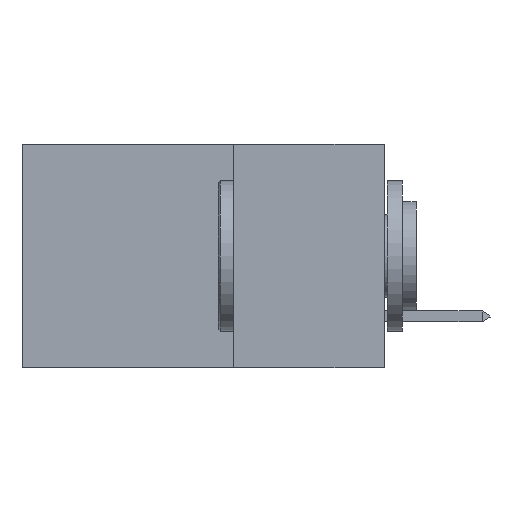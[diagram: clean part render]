
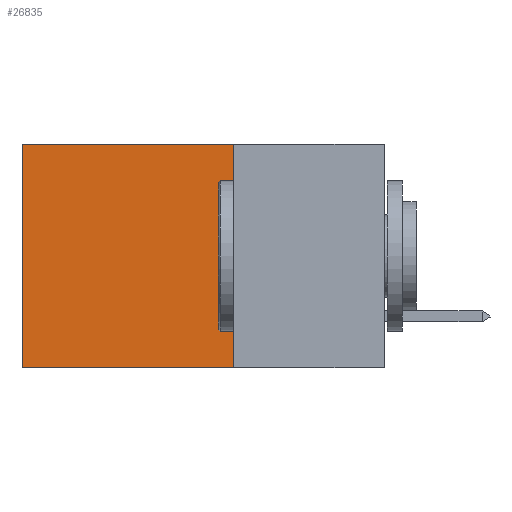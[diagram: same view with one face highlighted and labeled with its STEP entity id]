
A CAD part, left-side view. The second image highlights one B-rep face of the part: STEP entity #26835.
In plain terms, the highlighted planar face has unit normal (-1, 0, 0).
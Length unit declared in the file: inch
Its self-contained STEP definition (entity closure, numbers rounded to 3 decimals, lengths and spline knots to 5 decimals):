
#678 = LINE ( 'NONE', #2701, #26300 ) ;
#1016 = VECTOR ( 'NONE', #11773, 39.37008 ) ;
#2163 = EDGE_CURVE ( 'NONE', #8333, #25251, #678, .T. ) ;
#2221 = LINE ( 'NONE', #24124, #19066 ) ;
#2691 = DIRECTION ( 'NONE',  ( 0., 0., -1. ) ) ;
#2701 = CARTESIAN_POINT ( 'NONE',  ( 0.2875, 0.6, 0. ) ) ;
#3854 = CARTESIAN_POINT ( 'NONE',  ( 0.2875, 0.25, 0. ) ) ;
#5270 = DIRECTION ( 'NONE',  ( 0., 0., -1. ) ) ;
#5530 = EDGE_CURVE ( 'NONE', #25842, #25251, #10523, .T. ) ;
#7321 = ORIENTED_EDGE ( 'NONE', *, *, #14536, .T. ) ;
#8333 = VERTEX_POINT ( 'NONE', #20637 ) ;
#10315 = CARTESIAN_POINT ( 'NONE',  ( 0.2875, 0.25, -0.37 ) ) ;
#10523 = LINE ( 'NONE', #10315, #16123 ) ;
#11017 = ORIENTED_EDGE ( 'NONE', *, *, #5530, .F. ) ;
#11773 = DIRECTION ( 'NONE',  ( 0., 0., -1. ) ) ;
#12284 = AXIS2_PLACEMENT_3D ( 'NONE', #24380, #19585, #5270 ) ;
#12445 = CARTESIAN_POINT ( 'NONE',  ( 0.2875, 0.6, -0.37 ) ) ;
#14210 = ORIENTED_EDGE ( 'NONE', *, *, #2163, .T. ) ;
#14536 = EDGE_CURVE ( 'NONE', #19651, #8333, #2221, .T. ) ;
#15371 = ORIENTED_EDGE ( 'NONE', *, *, #29328, .F. ) ;
#16123 = VECTOR ( 'NONE', #24622, 39.37008 ) ;
#16455 = CARTESIAN_POINT ( 'NONE',  ( 0.2875, 0.25, 0. ) ) ;
#16977 = CARTESIAN_POINT ( 'NONE',  ( 0.2875, 0.25, -0.37 ) ) ;
#18849 = FACE_OUTER_BOUND ( 'NONE', #25481, .T. ) ;
#19066 = VECTOR ( 'NONE', #21678, 39.37008 ) ;
#19585 = DIRECTION ( 'NONE',  ( 1., 0., 0. ) ) ;
#19651 = VERTEX_POINT ( 'NONE', #3854 ) ;
#20637 = CARTESIAN_POINT ( 'NONE',  ( 0.2875, 0.6, 0. ) ) ;
#21678 = DIRECTION ( 'NONE',  ( 0., 1., 0. ) ) ;
#24124 = CARTESIAN_POINT ( 'NONE',  ( 0.2875, 0.25, 0. ) ) ;
#24380 = CARTESIAN_POINT ( 'NONE',  ( 0.2875, 0.25, 0. ) ) ;
#24622 = DIRECTION ( 'NONE',  ( 0., 1., 0. ) ) ;
#25251 = VERTEX_POINT ( 'NONE', #12445 ) ;
#25481 = EDGE_LOOP ( 'NONE', ( #14210, #11017, #15371, #7321 ) ) ;
#25842 = VERTEX_POINT ( 'NONE', #16977 ) ;
#26300 = VECTOR ( 'NONE', #2691, 39.37008 ) ;
#26597 = LINE ( 'NONE', #16455, #1016 ) ;
#26835 = ADVANCED_FACE ( 'NONE', ( #18849 ), #29139, .F. ) ;
#29139 = PLANE ( 'NONE',  #12284 ) ;
#29328 = EDGE_CURVE ( 'NONE', #19651, #25842, #26597, .T. ) ;
